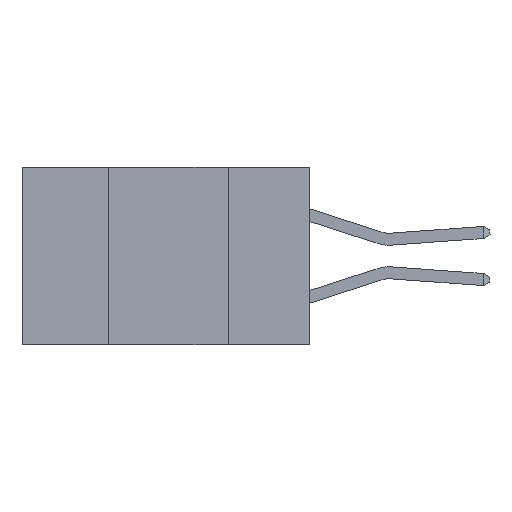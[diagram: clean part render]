
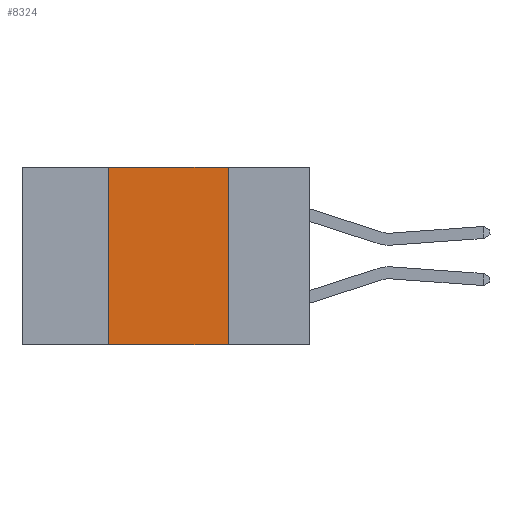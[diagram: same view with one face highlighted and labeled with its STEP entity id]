
A CAD part, left-side view. The second image highlights one B-rep face of the part: STEP entity #8324.
In plain terms, the highlighted planar face has unit normal (-1, 0, 0).
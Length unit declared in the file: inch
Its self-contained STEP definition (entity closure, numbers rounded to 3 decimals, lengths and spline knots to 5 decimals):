
#73 = DIRECTION ( 'NONE',  ( 0., 0., -1. ) ) ;
#269 = FACE_OUTER_BOUND ( 'NONE', #372, .T. ) ;
#372 = EDGE_LOOP ( 'NONE', ( #10446, #555, #1509, #13399 ) ) ;
#555 = ORIENTED_EDGE ( 'NONE', *, *, #8737, .F. ) ;
#563 = PLANE ( 'NONE',  #9762 ) ;
#671 = LINE ( 'NONE', #10229, #11953 ) ;
#896 = VERTEX_POINT ( 'NONE', #5995 ) ;
#1445 = EDGE_CURVE ( 'NONE', #5927, #6645, #671, .T. ) ;
#1509 = ORIENTED_EDGE ( 'NONE', *, *, #13275, .F. ) ;
#2624 = VECTOR ( 'NONE', #8400, 39.37008 ) ;
#3620 = CARTESIAN_POINT ( 'NONE',  ( 0., 0.42, 0. ) ) ;
#4333 = CARTESIAN_POINT ( 'NONE',  ( 0., 0.17, -0.37 ) ) ;
#5927 = VERTEX_POINT ( 'NONE', #6801 ) ;
#5987 = VECTOR ( 'NONE', #9871, 39.37008 ) ;
#5995 = CARTESIAN_POINT ( 'NONE',  ( 0., 0.17, 0. ) ) ;
#6127 = DIRECTION ( 'NONE',  ( 0., -1., 0. ) ) ;
#6645 = VERTEX_POINT ( 'NONE', #4333 ) ;
#6801 = CARTESIAN_POINT ( 'NONE',  ( 0., 0.42, -0.37 ) ) ;
#7081 = DIRECTION ( 'NONE',  ( 1., 0., 0. ) ) ;
#8324 = ADVANCED_FACE ( 'NONE', ( #269 ), #563, .F. ) ;
#8400 = DIRECTION ( 'NONE',  ( 0., -1., 0. ) ) ;
#8737 = EDGE_CURVE ( 'NONE', #10784, #896, #11518, .T. ) ;
#9000 = CARTESIAN_POINT ( 'NONE',  ( 0., 0.6, 0. ) ) ;
#9259 = LINE ( 'NONE', #9880, #5987 ) ;
#9381 = EDGE_CURVE ( 'NONE', #896, #6645, #9259, .T. ) ;
#9762 = AXIS2_PLACEMENT_3D ( 'NONE', #13261, #7081, #73 ) ;
#9871 = DIRECTION ( 'NONE',  ( 0., 0., -1. ) ) ;
#9880 = CARTESIAN_POINT ( 'NONE',  ( 0., 0.17, 0. ) ) ;
#10038 = DIRECTION ( 'NONE',  ( 0., 0., 1. ) ) ;
#10229 = CARTESIAN_POINT ( 'NONE',  ( 0., 0.6, -0.37 ) ) ;
#10446 = ORIENTED_EDGE ( 'NONE', *, *, #9381, .F. ) ;
#10784 = VERTEX_POINT ( 'NONE', #3620 ) ;
#11237 = VECTOR ( 'NONE', #10038, 39.37008 ) ;
#11518 = LINE ( 'NONE', #9000, #2624 ) ;
#11953 = VECTOR ( 'NONE', #6127, 39.37008 ) ;
#12171 = CARTESIAN_POINT ( 'NONE',  ( 0., 0.42, 0. ) ) ;
#12633 = LINE ( 'NONE', #12171, #11237 ) ;
#13261 = CARTESIAN_POINT ( 'NONE',  ( 0., 0.6, 0. ) ) ;
#13275 = EDGE_CURVE ( 'NONE', #5927, #10784, #12633, .T. ) ;
#13399 = ORIENTED_EDGE ( 'NONE', *, *, #1445, .T. ) ;
